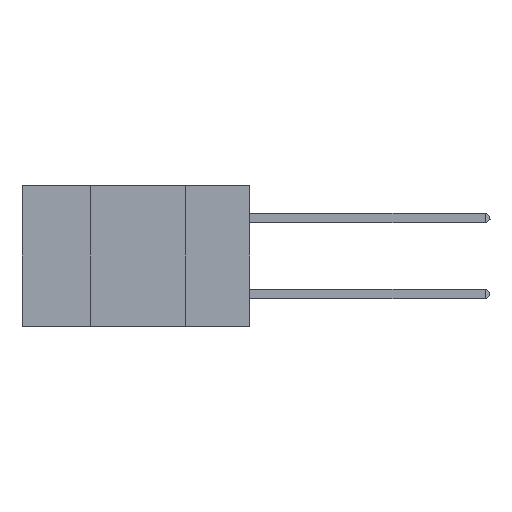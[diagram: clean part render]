
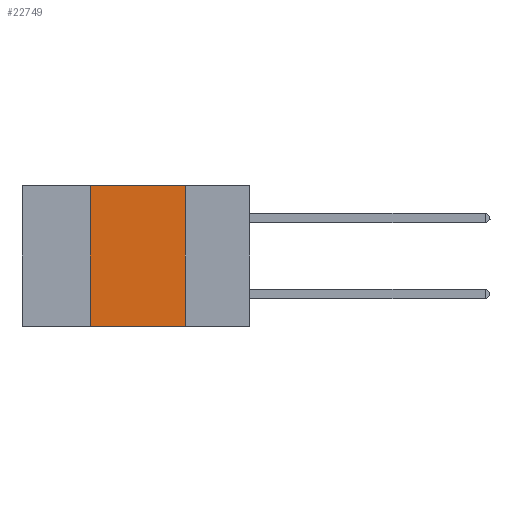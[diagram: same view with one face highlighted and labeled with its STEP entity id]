
A CAD part, left-side view. The second image highlights one B-rep face of the part: STEP entity #22749.
In plain terms, the highlighted planar face has unit normal (-1, 0, 0).
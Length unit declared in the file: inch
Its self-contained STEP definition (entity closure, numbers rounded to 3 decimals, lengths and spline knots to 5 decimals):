
#195 = CARTESIAN_POINT ( 'NONE',  ( 0., 0.6, 0. ) ) ;
#1319 = EDGE_CURVE ( 'NONE', #37590, #29125, #19577, .T. ) ;
#1596 = VERTEX_POINT ( 'NONE', #33831 ) ;
#2924 = LINE ( 'NONE', #29606, #36039 ) ;
#3530 = EDGE_CURVE ( 'NONE', #11175, #29125, #11147, .T. ) ;
#5282 = ORIENTED_EDGE ( 'NONE', *, *, #1319, .T. ) ;
#5384 = AXIS2_PLACEMENT_3D ( 'NONE', #19972, #19399, #16438 ) ;
#7462 = ORIENTED_EDGE ( 'NONE', *, *, #3530, .F. ) ;
#8440 = EDGE_CURVE ( 'NONE', #1596, #11175, #27074, .T. ) ;
#11147 = LINE ( 'NONE', #22350, #11761 ) ;
#11175 = VERTEX_POINT ( 'NONE', #32436 ) ;
#11761 = VECTOR ( 'NONE', #26067, 39.37008 ) ;
#14902 = DIRECTION ( 'NONE',  ( 0., -1., 0. ) ) ;
#16438 = DIRECTION ( 'NONE',  ( 0., 0., -1. ) ) ;
#16643 = EDGE_LOOP ( 'NONE', ( #7462, #38249, #17460, #5282 ) ) ;
#17460 = ORIENTED_EDGE ( 'NONE', *, *, #21105, .F. ) ;
#19399 = DIRECTION ( 'NONE',  ( 1., 0., 0. ) ) ;
#19577 = LINE ( 'NONE', #31534, #29719 ) ;
#19972 = CARTESIAN_POINT ( 'NONE',  ( 0., 0.6, 0. ) ) ;
#21105 = EDGE_CURVE ( 'NONE', #37590, #1596, #2924, .T. ) ;
#22328 = FACE_OUTER_BOUND ( 'NONE', #16643, .T. ) ;
#22350 = CARTESIAN_POINT ( 'NONE',  ( 0., 0.17, 0. ) ) ;
#22749 = ADVANCED_FACE ( 'NONE', ( #22328 ), #28987, .F. ) ;
#26067 = DIRECTION ( 'NONE',  ( 0., 0., -1. ) ) ;
#26420 = DIRECTION ( 'NONE',  ( 0., -1., 0. ) ) ;
#27074 = LINE ( 'NONE', #195, #29523 ) ;
#28987 = PLANE ( 'NONE',  #5384 ) ;
#29125 = VERTEX_POINT ( 'NONE', #32318 ) ;
#29523 = VECTOR ( 'NONE', #14902, 39.37008 ) ;
#29606 = CARTESIAN_POINT ( 'NONE',  ( 0., 0.42, 0. ) ) ;
#29719 = VECTOR ( 'NONE', #26420, 39.37008 ) ;
#29798 = DIRECTION ( 'NONE',  ( 0., 0., 1. ) ) ;
#31534 = CARTESIAN_POINT ( 'NONE',  ( 0., 0.6, -0.37 ) ) ;
#32318 = CARTESIAN_POINT ( 'NONE',  ( 0., 0.17, -0.37 ) ) ;
#32436 = CARTESIAN_POINT ( 'NONE',  ( 0., 0.17, 0. ) ) ;
#33831 = CARTESIAN_POINT ( 'NONE',  ( 0., 0.42, 0. ) ) ;
#36039 = VECTOR ( 'NONE', #29798, 39.37008 ) ;
#37590 = VERTEX_POINT ( 'NONE', #38428 ) ;
#38249 = ORIENTED_EDGE ( 'NONE', *, *, #8440, .F. ) ;
#38428 = CARTESIAN_POINT ( 'NONE',  ( 0., 0.42, -0.37 ) ) ;
